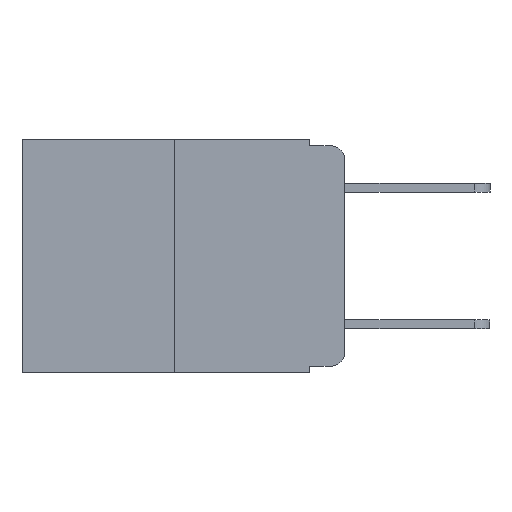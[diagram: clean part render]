
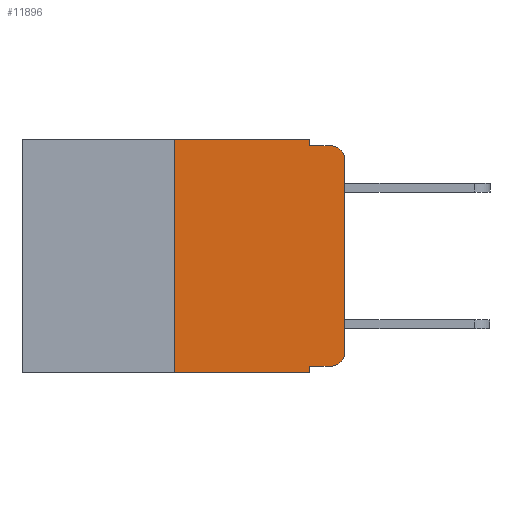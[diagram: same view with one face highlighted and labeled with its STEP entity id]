
A CAD part, left-side view. The second image highlights one B-rep face of the part: STEP entity #11896.
In plain terms, the highlighted planar face has unit normal (-1, 0, 0).
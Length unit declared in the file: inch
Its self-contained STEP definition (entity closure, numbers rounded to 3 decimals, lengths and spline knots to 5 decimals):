
#74 = CARTESIAN_POINT ( 'NONE',  ( 0., 0.25, 0. ) ) ;
#184 = CARTESIAN_POINT ( 'NONE',  ( 0., 0.051, -0.333 ) ) ;
#285 = ORIENTED_EDGE ( 'NONE', *, *, #12647, .T. ) ;
#306 = ORIENTED_EDGE ( 'NONE', *, *, #4521, .F. ) ;
#677 = ORIENTED_EDGE ( 'NONE', *, *, #6402, .F. ) ;
#1402 = DIRECTION ( 'NONE',  ( 0., 0., 1. ) ) ;
#1770 = CARTESIAN_POINT ( 'NONE',  ( 0., 0.473, -0.343 ) ) ;
#1938 = EDGE_LOOP ( 'NONE', ( #285, #2334, #677, #306, #9148, #7742, #8033, #6770, #7840, #3533 ) ) ;
#2254 = CARTESIAN_POINT ( 'NONE',  ( 0., 0.051, 0. ) ) ;
#2332 = CARTESIAN_POINT ( 'NONE',  ( 0., 0.02, -0.333 ) ) ;
#2334 = ORIENTED_EDGE ( 'NONE', *, *, #2885, .T. ) ;
#2484 = CARTESIAN_POINT ( 'NONE',  ( 0., 0.051, 0. ) ) ;
#2532 = VERTEX_POINT ( 'NONE', #184 ) ;
#2885 = EDGE_CURVE ( 'NONE', #4727, #4890, #11989, .T. ) ;
#3009 = CARTESIAN_POINT ( 'NONE',  ( 0., 0.473, 0. ) ) ;
#3244 = VERTEX_POINT ( 'NONE', #12130 ) ;
#3366 = CARTESIAN_POINT ( 'NONE',  ( 0., 0.051, -0.01 ) ) ;
#3533 = ORIENTED_EDGE ( 'NONE', *, *, #5446, .T. ) ;
#3555 = VERTEX_POINT ( 'NONE', #2332 ) ;
#3949 = VECTOR ( 'NONE', #11296, 39.37008 ) ;
#3988 = AXIS2_PLACEMENT_3D ( 'NONE', #4023, #11045, #5057 ) ;
#4023 = CARTESIAN_POINT ( 'NONE',  ( 0., 0.02, -0.313 ) ) ;
#4099 = CARTESIAN_POINT ( 'NONE',  ( 0., 0.25, -0.343 ) ) ;
#4251 = AXIS2_PLACEMENT_3D ( 'NONE', #3009, #13147, #7188 ) ;
#4384 = LINE ( 'NONE', #3366, #11763 ) ;
#4521 = EDGE_CURVE ( 'NONE', #3244, #5172, #6688, .T. ) ;
#4636 = CARTESIAN_POINT ( 'NONE',  ( 0., 0.051, -0.01 ) ) ;
#4727 = VERTEX_POINT ( 'NONE', #8030 ) ;
#4890 = VERTEX_POINT ( 'NONE', #12343 ) ;
#5057 = DIRECTION ( 'NONE',  ( 0., 0., -1. ) ) ;
#5172 = VERTEX_POINT ( 'NONE', #4636 ) ;
#5219 = CARTESIAN_POINT ( 'NONE',  ( 0., 0.473, 0. ) ) ;
#5242 = VECTOR ( 'NONE', #8776, 39.37008 ) ;
#5445 = VERTEX_POINT ( 'NONE', #7066 ) ;
#5446 = EDGE_CURVE ( 'NONE', #3555, #6091, #11448, .T. ) ;
#5578 = LINE ( 'NONE', #10730, #5242 ) ;
#5789 = FACE_OUTER_BOUND ( 'NONE', #1938, .T. ) ;
#6091 = VERTEX_POINT ( 'NONE', #8079 ) ;
#6402 = EDGE_CURVE ( 'NONE', #5172, #4890, #4384, .T. ) ;
#6688 = LINE ( 'NONE', #2254, #3949 ) ;
#6770 = ORIENTED_EDGE ( 'NONE', *, *, #12105, .F. ) ;
#6875 = DIRECTION ( 'NONE',  ( 0., 0., -1. ) ) ;
#7044 = DIRECTION ( 'NONE',  ( 0., 0., 1. ) ) ;
#7066 = CARTESIAN_POINT ( 'NONE',  ( 0., 0.051, -0.343 ) ) ;
#7171 = VECTOR ( 'NONE', #1402, 39.37008 ) ;
#7188 = DIRECTION ( 'NONE',  ( 0., 0., -1. ) ) ;
#7274 = EDGE_CURVE ( 'NONE', #10080, #12135, #13333, .T. ) ;
#7321 = VECTOR ( 'NONE', #9076, 39.37008 ) ;
#7348 = DIRECTION ( 'NONE',  ( -1., 0., 0. ) ) ;
#7387 = CARTESIAN_POINT ( 'NONE',  ( 0., 0.02, -0.03 ) ) ;
#7742 = ORIENTED_EDGE ( 'NONE', *, *, #7274, .F. ) ;
#7790 = CARTESIAN_POINT ( 'NONE',  ( 0., 0., 0. ) ) ;
#7840 = ORIENTED_EDGE ( 'NONE', *, *, #13070, .T. ) ;
#8030 = CARTESIAN_POINT ( 'NONE',  ( 0., 0., -0.03 ) ) ;
#8033 = ORIENTED_EDGE ( 'NONE', *, *, #12769, .T. ) ;
#8079 = CARTESIAN_POINT ( 'NONE',  ( 0., 0., -0.313 ) ) ;
#8675 = VECTOR ( 'NONE', #10204, 39.37008 ) ;
#8677 = DIRECTION ( 'NONE',  ( 0., 0., -1. ) ) ;
#8776 = DIRECTION ( 'NONE',  ( 0., -1., 0. ) ) ;
#8976 = LINE ( 'NONE', #5219, #8675 ) ;
#9076 = DIRECTION ( 'NONE',  ( 0., -1., 0. ) ) ;
#9148 = ORIENTED_EDGE ( 'NONE', *, *, #10166, .F. ) ;
#9669 = VECTOR ( 'NONE', #8677, 39.37008 ) ;
#9949 = LINE ( 'NONE', #1770, #7321 ) ;
#9959 = AXIS2_PLACEMENT_3D ( 'NONE', #7387, #7348, #6875 ) ;
#10080 = VERTEX_POINT ( 'NONE', #4099 ) ;
#10123 = PLANE ( 'NONE',  #4251 ) ;
#10166 = EDGE_CURVE ( 'NONE', #12135, #3244, #8976, .T. ) ;
#10204 = DIRECTION ( 'NONE',  ( 0., -1., 0. ) ) ;
#10730 = CARTESIAN_POINT ( 'NONE',  ( 0., 0.051, -0.333 ) ) ;
#11045 = DIRECTION ( 'NONE',  ( -1., 0., 0. ) ) ;
#11296 = DIRECTION ( 'NONE',  ( 0., 0., -1. ) ) ;
#11448 = CIRCLE ( 'NONE', #3988, 0.02 ) ;
#11763 = VECTOR ( 'NONE', #12410, 39.37008 ) ;
#11896 = ADVANCED_FACE ( 'NONE', ( #5789 ), #10123, .F. ) ;
#11989 = CIRCLE ( 'NONE', #9959, 0.02 ) ;
#12105 = EDGE_CURVE ( 'NONE', #2532, #5445, #12330, .T. ) ;
#12130 = CARTESIAN_POINT ( 'NONE',  ( 0., 0.051, 0. ) ) ;
#12135 = VERTEX_POINT ( 'NONE', #74 ) ;
#12151 = LINE ( 'NONE', #7790, #7171 ) ;
#12330 = LINE ( 'NONE', #2484, #9669 ) ;
#12343 = CARTESIAN_POINT ( 'NONE',  ( 0., 0.02, -0.01 ) ) ;
#12410 = DIRECTION ( 'NONE',  ( 0., -1., 0. ) ) ;
#12647 = EDGE_CURVE ( 'NONE', #6091, #4727, #12151, .T. ) ;
#12769 = EDGE_CURVE ( 'NONE', #10080, #5445, #9949, .T. ) ;
#13002 = CARTESIAN_POINT ( 'NONE',  ( 0., 0.25, 0. ) ) ;
#13007 = VECTOR ( 'NONE', #7044, 39.37008 ) ;
#13070 = EDGE_CURVE ( 'NONE', #2532, #3555, #5578, .T. ) ;
#13147 = DIRECTION ( 'NONE',  ( 1., 0., 0. ) ) ;
#13333 = LINE ( 'NONE', #13002, #13007 ) ;
